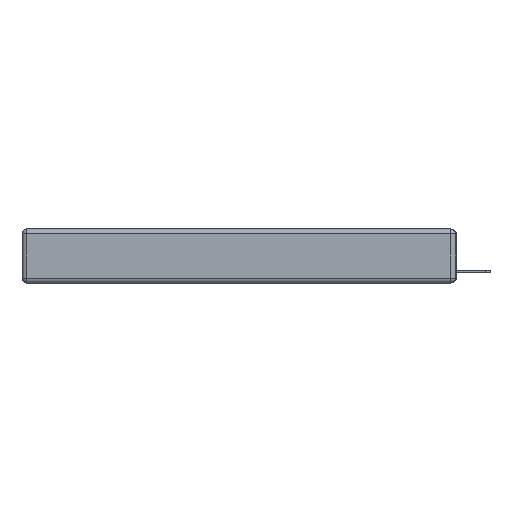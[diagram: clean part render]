
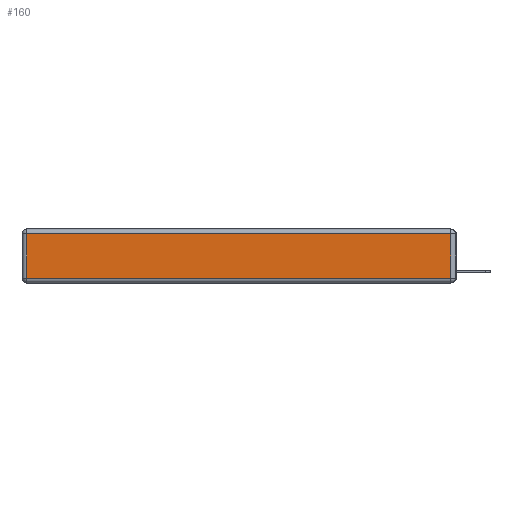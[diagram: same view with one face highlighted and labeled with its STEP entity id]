
A CAD part, left-side view. The second image highlights one B-rep face of the part: STEP entity #160.
In plain terms, the highlighted planar face has unit normal (-1, 0, 0).
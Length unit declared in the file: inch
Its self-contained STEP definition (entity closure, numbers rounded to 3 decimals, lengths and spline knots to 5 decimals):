
#105 = CARTESIAN_POINT ( 'NONE',  ( 0., 0.03, -0.313 ) ) ;
#160 = ADVANCED_FACE ( 'NONE', ( #7036 ), #5553, .T. ) ;
#774 = VERTEX_POINT ( 'NONE', #7901 ) ;
#977 = ORIENTED_EDGE ( 'NONE', *, *, #9958, .T. ) ;
#1199 = DIRECTION ( 'NONE',  ( 0., 1., 0. ) ) ;
#1281 = CARTESIAN_POINT ( 'NONE',  ( 0., 2.75, -0.03 ) ) ;
#1478 = LINE ( 'NONE', #1281, #8838 ) ;
#1714 = DIRECTION ( 'NONE',  ( -1., 0., 0. ) ) ;
#2107 = ORIENTED_EDGE ( 'NONE', *, *, #24770, .T. ) ;
#3439 = AXIS2_PLACEMENT_3D ( 'NONE', #11323, #1714, #9441 ) ;
#3990 = CARTESIAN_POINT ( 'NONE',  ( 0., 0., -0.313 ) ) ;
#4052 = LINE ( 'NONE', #3990, #7133 ) ;
#5553 = PLANE ( 'NONE',  #3439 ) ;
#7036 = FACE_OUTER_BOUND ( 'NONE', #13311, .T. ) ;
#7133 = VECTOR ( 'NONE', #15276, 39.37008 ) ;
#7495 = CARTESIAN_POINT ( 'NONE',  ( 0., 2.72, -0.343 ) ) ;
#7901 = CARTESIAN_POINT ( 'NONE',  ( 0., 2.72, -0.03 ) ) ;
#8302 = EDGE_CURVE ( 'NONE', #12164, #22550, #21745, .T. ) ;
#8838 = VECTOR ( 'NONE', #1199, 39.37008 ) ;
#8946 = EDGE_CURVE ( 'NONE', #21841, #12164, #4052, .T. ) ;
#9040 = ORIENTED_EDGE ( 'NONE', *, *, #8946, .T. ) ;
#9246 = DIRECTION ( 'NONE',  ( 0., 0., 1. ) ) ;
#9441 = DIRECTION ( 'NONE',  ( 0., 0., 1. ) ) ;
#9533 = CARTESIAN_POINT ( 'NONE',  ( 0., 0.03, -0.03 ) ) ;
#9958 = EDGE_CURVE ( 'NONE', #774, #21841, #10749, .T. ) ;
#10749 = LINE ( 'NONE', #7495, #23826 ) ;
#11323 = CARTESIAN_POINT ( 'NONE',  ( 0., 0., -0.343 ) ) ;
#11413 = ORIENTED_EDGE ( 'NONE', *, *, #8302, .T. ) ;
#12164 = VERTEX_POINT ( 'NONE', #105 ) ;
#13311 = EDGE_LOOP ( 'NONE', ( #9040, #11413, #2107, #977 ) ) ;
#15276 = DIRECTION ( 'NONE',  ( 0., -1., 0. ) ) ;
#20652 = CARTESIAN_POINT ( 'NONE',  ( 0., 2.72, -0.313 ) ) ;
#20845 = DIRECTION ( 'NONE',  ( 0., 0., -1. ) ) ;
#21745 = LINE ( 'NONE', #25058, #22676 ) ;
#21841 = VERTEX_POINT ( 'NONE', #20652 ) ;
#22550 = VERTEX_POINT ( 'NONE', #9533 ) ;
#22676 = VECTOR ( 'NONE', #9246, 39.37008 ) ;
#23826 = VECTOR ( 'NONE', #20845, 39.37008 ) ;
#24770 = EDGE_CURVE ( 'NONE', #22550, #774, #1478, .T. ) ;
#25058 = CARTESIAN_POINT ( 'NONE',  ( 0., 0.03, -0.343 ) ) ;
